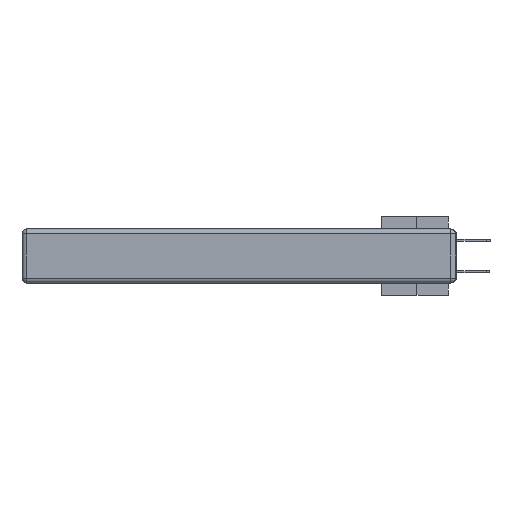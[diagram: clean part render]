
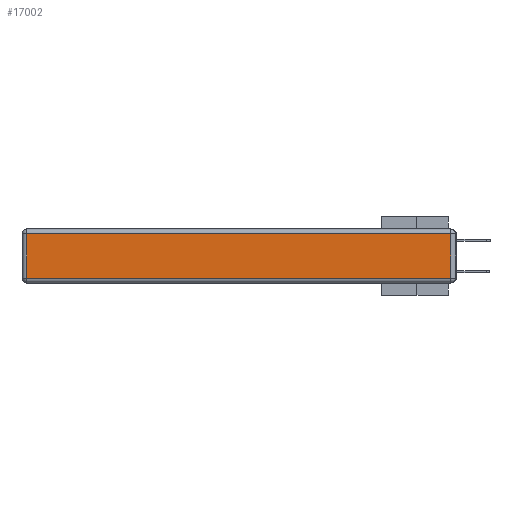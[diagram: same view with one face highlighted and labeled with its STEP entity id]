
A CAD part, left-side view. The second image highlights one B-rep face of the part: STEP entity #17002.
In plain terms, the highlighted planar face has unit normal (-1, 0, 0).
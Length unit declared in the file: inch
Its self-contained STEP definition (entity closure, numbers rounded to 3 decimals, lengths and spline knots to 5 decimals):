
#128 = CARTESIAN_POINT ( 'NONE',  ( 0., 2.72, -0.343 ) ) ;
#1762 = DIRECTION ( 'NONE',  ( 0., 1., 0. ) ) ;
#3112 = VECTOR ( 'NONE', #25730, 39.37008 ) ;
#3614 = CARTESIAN_POINT ( 'NONE',  ( 0., 0.03, -0.343 ) ) ;
#3738 = CARTESIAN_POINT ( 'NONE',  ( 0., 0.03, -0.313 ) ) ;
#4823 = CARTESIAN_POINT ( 'NONE',  ( 0., 2.75, -0.03 ) ) ;
#5766 = CARTESIAN_POINT ( 'NONE',  ( 0., 0., -0.313 ) ) ;
#5777 = CARTESIAN_POINT ( 'NONE',  ( 0., 2.72, -0.03 ) ) ;
#6273 = CARTESIAN_POINT ( 'NONE',  ( 0., 0.03, -0.03 ) ) ;
#7280 = AXIS2_PLACEMENT_3D ( 'NONE', #8039, #8275, #27522 ) ;
#7531 = EDGE_LOOP ( 'NONE', ( #21304, #26292, #26062, #16983 ) ) ;
#8039 = CARTESIAN_POINT ( 'NONE',  ( 0., 0., -0.343 ) ) ;
#8275 = DIRECTION ( 'NONE',  ( -1., 0., 0. ) ) ;
#8483 = EDGE_CURVE ( 'NONE', #32223, #31767, #32046, .T. ) ;
#9741 = FACE_OUTER_BOUND ( 'NONE', #7531, .T. ) ;
#11393 = LINE ( 'NONE', #3614, #3112 ) ;
#12617 = LINE ( 'NONE', #128, #26352 ) ;
#16983 = ORIENTED_EDGE ( 'NONE', *, *, #26620, .T. ) ;
#17002 = ADVANCED_FACE ( 'NONE', ( #9741 ), #35725, .T. ) ;
#18587 = VECTOR ( 'NONE', #1762, 39.37008 ) ;
#18950 = EDGE_CURVE ( 'NONE', #31767, #30564, #11393, .T. ) ;
#19397 = CARTESIAN_POINT ( 'NONE',  ( 0., 2.72, -0.313 ) ) ;
#21304 = ORIENTED_EDGE ( 'NONE', *, *, #8483, .T. ) ;
#22349 = DIRECTION ( 'NONE',  ( 0., 0., -1. ) ) ;
#22359 = DIRECTION ( 'NONE',  ( 0., -1., 0. ) ) ;
#24720 = VECTOR ( 'NONE', #22359, 39.37008 ) ;
#25730 = DIRECTION ( 'NONE',  ( 0., 0., 1. ) ) ;
#26062 = ORIENTED_EDGE ( 'NONE', *, *, #26410, .T. ) ;
#26292 = ORIENTED_EDGE ( 'NONE', *, *, #18950, .T. ) ;
#26352 = VECTOR ( 'NONE', #22349, 39.37008 ) ;
#26410 = EDGE_CURVE ( 'NONE', #30564, #30445, #33289, .T. ) ;
#26620 = EDGE_CURVE ( 'NONE', #30445, #32223, #12617, .T. ) ;
#27522 = DIRECTION ( 'NONE',  ( 0., 0., 1. ) ) ;
#30445 = VERTEX_POINT ( 'NONE', #5777 ) ;
#30564 = VERTEX_POINT ( 'NONE', #6273 ) ;
#31767 = VERTEX_POINT ( 'NONE', #3738 ) ;
#32046 = LINE ( 'NONE', #5766, #24720 ) ;
#32223 = VERTEX_POINT ( 'NONE', #19397 ) ;
#33289 = LINE ( 'NONE', #4823, #18587 ) ;
#35725 = PLANE ( 'NONE',  #7280 ) ;
